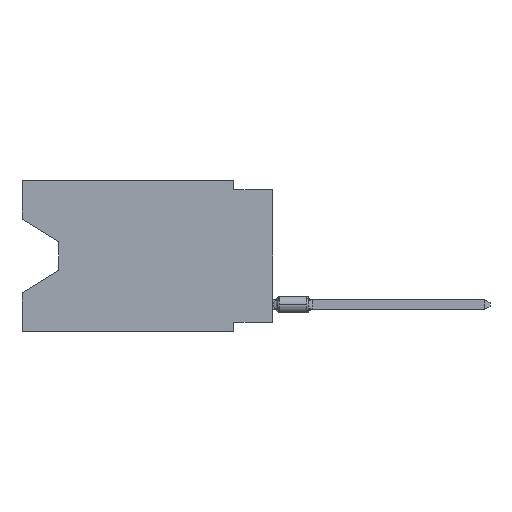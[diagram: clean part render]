
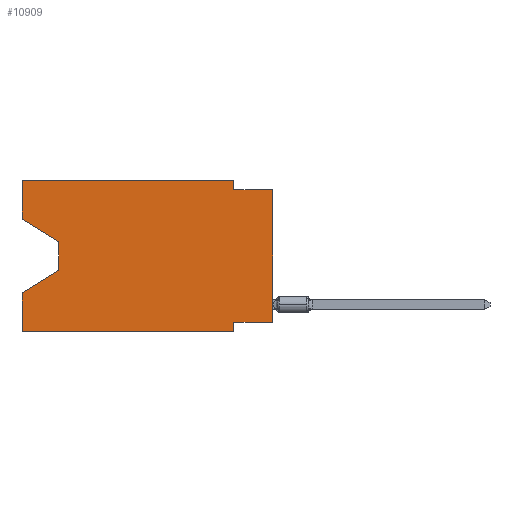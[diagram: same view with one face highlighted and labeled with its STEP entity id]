
A CAD part, left-side view. The second image highlights one B-rep face of the part: STEP entity #10909.
In plain terms, the highlighted planar face has unit normal (-1, 0, 0).
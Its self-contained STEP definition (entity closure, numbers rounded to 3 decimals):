
#550 = EDGE_CURVE ( 'NONE', #3863, #11859, #11519, .T. ) ;
#721 = VERTEX_POINT ( 'NONE', #6741 ) ;
#1077 = VECTOR ( 'NONE', #7244, 1000. ) ;
#1476 = VERTEX_POINT ( 'NONE', #9885 ) ;
#2344 = ORIENTED_EDGE ( 'NONE', *, *, #14499, .F. ) ;
#2354 = CARTESIAN_POINT ( 'NONE',  ( 0., 2.54, -0.635 ) ) ;
#2915 = DIRECTION ( 'NONE',  ( 0., 0., 1. ) ) ;
#3712 = VECTOR ( 'NONE', #11862, 1000. ) ;
#3759 = VERTEX_POINT ( 'NONE', #6654 ) ;
#3810 = DIRECTION ( 'NONE',  ( 0., 1., 0. ) ) ;
#3863 = VERTEX_POINT ( 'NONE', #2354 ) ;
#4383 = CARTESIAN_POINT ( 'NONE',  ( 0., 16.383, -2.546 ) ) ;
#4382 = VECTOR ( 'NONE', #11083, 1000. ) ;
#4505 = VECTOR ( 'NONE', #15023, 1000. ) ;
#4598 = PLANE ( 'NONE',  #10213 ) ;
#4618 = VECTOR ( 'NONE', #2915, 1000. ) ;
#4886 = CARTESIAN_POINT ( 'NONE',  ( 0., 2.54, 0. ) ) ;
#4955 = LINE ( 'NONE', #11758, #3712 ) ;
#5639 = VERTEX_POINT ( 'NONE', #11604 ) ;
#5784 = EDGE_CURVE ( 'NONE', #5861, #10440, #15677, .T. ) ;
#5861 = VERTEX_POINT ( 'NONE', #18361 ) ;
#6149 = CARTESIAN_POINT ( 'NONE',  ( 0., 16.383, 0. ) ) ;
#6408 = ORIENTED_EDGE ( 'NONE', *, *, #18579, .F. ) ;
#6654 = CARTESIAN_POINT ( 'NONE',  ( 0., 2.54, -9.271 ) ) ;
#6741 = CARTESIAN_POINT ( 'NONE',  ( 0., 0., -9.271 ) ) ;
#7024 = CARTESIAN_POINT ( 'NONE',  ( 0., 0., -0.635 ) ) ;
#7244 = DIRECTION ( 'NONE',  ( 0., -1., 0. ) ) ;
#7288 = CARTESIAN_POINT ( 'NONE',  ( 0., 16.383, -2.546 ) ) ;
#7892 = ORIENTED_EDGE ( 'NONE', *, *, #13570, .T. ) ;
#8011 = VECTOR ( 'NONE', #18146, 1000. ) ;
#8333 = VERTEX_POINT ( 'NONE', #6149 ) ;
#8452 = DIRECTION ( 'NONE',  ( 0., 0., -1. ) ) ;
#9152 = ORIENTED_EDGE ( 'NONE', *, *, #15138, .T. ) ;
#9217 = EDGE_CURVE ( 'NONE', #9999, #3863, #13897, .T. ) ;
#9356 = ORIENTED_EDGE ( 'NONE', *, *, #9217, .F. ) ;
#9649 = LINE ( 'NONE', #13265, #8011 ) ;
#9875 = EDGE_CURVE ( 'NONE', #5639, #1476, #9649, .T. ) ;
#9885 = CARTESIAN_POINT ( 'NONE',  ( 0., 16.383, -7.36 ) ) ;
#9999 = VERTEX_POINT ( 'NONE', #4886 ) ;
#10062 = CARTESIAN_POINT ( 'NONE',  ( 0., 13.97, -5.893 ) ) ;
#10213 = AXIS2_PLACEMENT_3D ( 'NONE', #18536, #18411, #13318 ) ;
#10287 = ORIENTED_EDGE ( 'NONE', *, *, #19551, .F. ) ;
#10327 = EDGE_CURVE ( 'NONE', #8333, #9999, #12588, .T. ) ;
#10440 = VERTEX_POINT ( 'NONE', #10062 ) ;
#10909 = ADVANCED_FACE ( 'NONE', ( #13220 ), #4598, .F. ) ;
#11083 = DIRECTION ( 'NONE',  ( 0., -0.855, -0.519 ) ) ;
#11259 = VECTOR ( 'NONE', #20533, 1000. ) ;
#11287 = ORIENTED_EDGE ( 'NONE', *, *, #9875, .F. ) ;
#11519 = LINE ( 'NONE', #15853, #1077 ) ;
#11604 = CARTESIAN_POINT ( 'NONE',  ( 0., 16.383, -9.906 ) ) ;
#11758 = CARTESIAN_POINT ( 'NONE',  ( 0., 16.383, -9.906 ) ) ;
#11799 = DIRECTION ( 'NONE',  ( 0., 0.855, -0.519 ) ) ;
#11859 = VERTEX_POINT ( 'NONE', #7024 ) ;
#11862 = DIRECTION ( 'NONE',  ( 0., -1., 0. ) ) ;
#12024 = VECTOR ( 'NONE', #12260, 1000. ) ;
#12038 = EDGE_CURVE ( 'NONE', #5639, #19656, #4955, .T. ) ;
#12064 = ORIENTED_EDGE ( 'NONE', *, *, #16925, .T. ) ;
#12260 = DIRECTION ( 'NONE',  ( 0., 0., -1. ) ) ;
#12588 = LINE ( 'NONE', #14724, #15600 ) ;
#12675 = ORIENTED_EDGE ( 'NONE', *, *, #12038, .T. ) ;
#13220 = FACE_OUTER_BOUND ( 'NONE', #20370, .T. ) ;
#13265 = CARTESIAN_POINT ( 'NONE',  ( 0., 16.383, 0. ) ) ;
#13318 = DIRECTION ( 'NONE',  ( 0., 0., -1. ) ) ;
#13570 = EDGE_CURVE ( 'NONE', #16566, #5861, #17874, .T. ) ;
#13621 = LINE ( 'NONE', #15100, #11259 ) ;
#13897 = LINE ( 'NONE', #22383, #22404 ) ;
#14499 = EDGE_CURVE ( 'NONE', #721, #3759, #17519, .T. ) ;
#14724 = CARTESIAN_POINT ( 'NONE',  ( 0., 16.383, 0. ) ) ;
#14917 = CARTESIAN_POINT ( 'NONE',  ( 0., 2.54, -9.906 ) ) ;
#15023 = DIRECTION ( 'NONE',  ( 0., 0., -1. ) ) ;
#15100 = CARTESIAN_POINT ( 'NONE',  ( 0., 0., 0. ) ) ;
#15138 = EDGE_CURVE ( 'NONE', #721, #11859, #13621, .T. ) ;
#15207 = LINE ( 'NONE', #15436, #21302 ) ;
#15256 = CARTESIAN_POINT ( 'NONE',  ( 0., 16.383, 0. ) ) ;
#15436 = CARTESIAN_POINT ( 'NONE',  ( 0., 13.97, -5.893 ) ) ;
#15600 = VECTOR ( 'NONE', #21738, 1000. ) ;
#15677 = LINE ( 'NONE', #15775, #12024 ) ;
#15775 = CARTESIAN_POINT ( 'NONE',  ( 0., 13.97, -4.013 ) ) ;
#15853 = CARTESIAN_POINT ( 'NONE',  ( 0., 0., -0.635 ) ) ;
#16311 = ORIENTED_EDGE ( 'NONE', *, *, #5784, .T. ) ;
#16350 = VECTOR ( 'NONE', #3810, 1000. ) ;
#16566 = VERTEX_POINT ( 'NONE', #7288 ) ;
#16925 = EDGE_CURVE ( 'NONE', #10440, #1476, #15207, .T. ) ;
#17519 = LINE ( 'NONE', #21036, #16350 ) ;
#17874 = LINE ( 'NONE', #4383, #4382 ) ;
#18146 = DIRECTION ( 'NONE',  ( 0., 0., 1. ) ) ;
#18361 = CARTESIAN_POINT ( 'NONE',  ( 0., 13.97, -4.013 ) ) ;
#18411 = DIRECTION ( 'NONE',  ( 1., 0., 0. ) ) ;
#18536 = CARTESIAN_POINT ( 'NONE',  ( 0., 16.383, 0. ) ) ;
#18579 = EDGE_CURVE ( 'NONE', #16566, #8333, #22272, .T. ) ;
#18771 = ORIENTED_EDGE ( 'NONE', *, *, #10327, .F. ) ;
#19551 = EDGE_CURVE ( 'NONE', #3759, #19656, #22151, .T. ) ;
#19656 = VERTEX_POINT ( 'NONE', #14917 ) ;
#20115 = CARTESIAN_POINT ( 'NONE',  ( 0., 2.54, -9.906 ) ) ;
#20370 = EDGE_LOOP ( 'NONE', ( #7892, #16311, #12064, #11287, #12675, #10287, #2344, #9152, #22183, #9356, #18771, #6408 ) ) ;
#20533 = DIRECTION ( 'NONE',  ( 0., 0., 1. ) ) ;
#21036 = CARTESIAN_POINT ( 'NONE',  ( 0., 0., -9.271 ) ) ;
#21302 = VECTOR ( 'NONE', #11799, 1000. ) ;
#21738 = DIRECTION ( 'NONE',  ( 0., -1., 0. ) ) ;
#22151 = LINE ( 'NONE', #20115, #4505 ) ;
#22183 = ORIENTED_EDGE ( 'NONE', *, *, #550, .F. ) ;
#22272 = LINE ( 'NONE', #15256, #4618 ) ;
#22383 = CARTESIAN_POINT ( 'NONE',  ( 0., 2.54, 0. ) ) ;
#22404 = VECTOR ( 'NONE', #8452, 1000. ) ;
